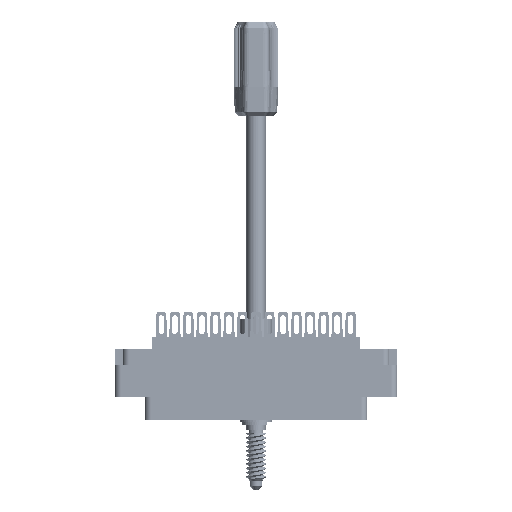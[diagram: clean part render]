
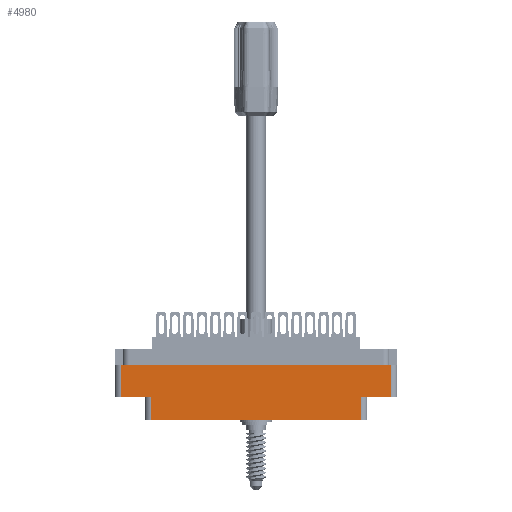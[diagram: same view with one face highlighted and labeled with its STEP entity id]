
A CAD part, front view. The second image highlights one B-rep face of the part: STEP entity #4980.
In plain terms, the highlighted planar face has unit normal (0, -1, 0).
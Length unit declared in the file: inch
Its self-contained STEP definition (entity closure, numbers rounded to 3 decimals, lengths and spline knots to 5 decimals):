
#68 = AXIS2_PLACEMENT_3D ( 'NONE', #38660, #51756, #12923 ) ;
#1185 = ORIENTED_EDGE ( 'NONE', *, *, #69164, .F. ) ;
#2698 = EDGE_CURVE ( 'NONE', #15390, #13735, #11628, .T. ) ;
#2727 = EDGE_CURVE ( 'NONE', #13735, #22982, #65832, .T. ) ;
#4980 = ADVANCED_FACE ( 'NONE', ( #72628 ), #77641, .T. ) ;
#5474 = CARTESIAN_POINT ( 'NONE',  ( 1.006, -0.617, -0.578 ) ) ;
#6226 = DIRECTION ( 'NONE',  ( 0., 0., -1. ) ) ;
#6946 = ORIENTED_EDGE ( 'NONE', *, *, #21479, .T. ) ;
#10073 = EDGE_CURVE ( 'NONE', #69673, #34776, #63557, .T. ) ;
#10220 = CARTESIAN_POINT ( 'NONE',  ( 0., -0.617, -0.578 ) ) ;
#10474 = ORIENTED_EDGE ( 'NONE', *, *, #2698, .T. ) ;
#11628 = LINE ( 'NONE', #51488, #83118 ) ;
#12923 = DIRECTION ( 'NONE',  ( 0., 0., -1. ) ) ;
#13735 = VERTEX_POINT ( 'NONE', #47508 ) ;
#15390 = VERTEX_POINT ( 'NONE', #29045 ) ;
#19813 = CARTESIAN_POINT ( 'NONE',  ( 0., -0.617, -0.578 ) ) ;
#21479 = EDGE_CURVE ( 'NONE', #49204, #60126, #30562, .T. ) ;
#21602 = ORIENTED_EDGE ( 'NONE', *, *, #44394, .F. ) ;
#22130 = LINE ( 'NONE', #24804, #57934 ) ;
#22982 = VERTEX_POINT ( 'NONE', #35612 ) ;
#24804 = CARTESIAN_POINT ( 'NONE',  ( 0., -0.617, -0.274 ) ) ;
#25062 = VECTOR ( 'NONE', #6226, 39.37008 ) ;
#27224 = DIRECTION ( 'NONE',  ( -1., 0., 0. ) ) ;
#28212 = CARTESIAN_POINT ( 'NONE',  ( -1.006, -0.617, -0.798 ) ) ;
#29045 = CARTESIAN_POINT ( 'NONE',  ( -1.006, -0.617, -0.798 ) ) ;
#29663 = CARTESIAN_POINT ( 'NONE',  ( -1.297, -0.617, -0.274 ) ) ;
#30562 = LINE ( 'NONE', #10220, #45898 ) ;
#31594 = CARTESIAN_POINT ( 'NONE',  ( 1.297, -0.617, -0.274 ) ) ;
#31770 = VECTOR ( 'NONE', #79518, 39.37008 ) ;
#34033 = ORIENTED_EDGE ( 'NONE', *, *, #10073, .T. ) ;
#34776 = VERTEX_POINT ( 'NONE', #31594 ) ;
#35612 = CARTESIAN_POINT ( 'NONE',  ( 1.006, -0.617, -0.578 ) ) ;
#36722 = EDGE_LOOP ( 'NONE', ( #6946, #54830, #10474, #54891, #1185, #34033, #21602, #52763 ) ) ;
#38660 = CARTESIAN_POINT ( 'NONE',  ( -1.359, -0.617, -0.798 ) ) ;
#42337 = VECTOR ( 'NONE', #58096, 39.37008 ) ;
#44394 = EDGE_CURVE ( 'NONE', #64825, #34776, #22130, .T. ) ;
#45319 = EDGE_CURVE ( 'NONE', #64825, #49204, #53655, .T. ) ;
#45898 = VECTOR ( 'NONE', #82438, 39.37008 ) ;
#47508 = CARTESIAN_POINT ( 'NONE',  ( 1.006, -0.617, -0.798 ) ) ;
#47764 = VECTOR ( 'NONE', #27224, 39.37008 ) ;
#49204 = VERTEX_POINT ( 'NONE', #56196 ) ;
#50012 = CARTESIAN_POINT ( 'NONE',  ( 1.297, -0.617, -0.798 ) ) ;
#51189 = DIRECTION ( 'NONE',  ( 1., 0., 0. ) ) ;
#51488 = CARTESIAN_POINT ( 'NONE',  ( -1.359, -0.617, -0.798 ) ) ;
#51756 = DIRECTION ( 'NONE',  ( 0., -1., 0. ) ) ;
#51900 = EDGE_CURVE ( 'NONE', #60126, #15390, #66513, .T. ) ;
#52763 = ORIENTED_EDGE ( 'NONE', *, *, #45319, .T. ) ;
#53655 = LINE ( 'NONE', #83906, #25062 ) ;
#54830 = ORIENTED_EDGE ( 'NONE', *, *, #51900, .T. ) ;
#54891 = ORIENTED_EDGE ( 'NONE', *, *, #2727, .T. ) ;
#56045 = DIRECTION ( 'NONE',  ( 0., 0., 1. ) ) ;
#56196 = CARTESIAN_POINT ( 'NONE',  ( -1.297, -0.617, -0.578 ) ) ;
#57925 = DIRECTION ( 'NONE',  ( 1., 0., 0. ) ) ;
#57934 = VECTOR ( 'NONE', #57925, 39.37008 ) ;
#58096 = DIRECTION ( 'NONE',  ( 0., 0., 1. ) ) ;
#60126 = VERTEX_POINT ( 'NONE', #78392 ) ;
#63557 = LINE ( 'NONE', #50012, #78738 ) ;
#64825 = VERTEX_POINT ( 'NONE', #29663 ) ;
#65832 = LINE ( 'NONE', #5474, #42337 ) ;
#66513 = LINE ( 'NONE', #28212, #31770 ) ;
#69164 = EDGE_CURVE ( 'NONE', #69673, #22982, #84369, .T. ) ;
#69673 = VERTEX_POINT ( 'NONE', #76102 ) ;
#72628 = FACE_OUTER_BOUND ( 'NONE', #36722, .T. ) ;
#76102 = CARTESIAN_POINT ( 'NONE',  ( 1.297, -0.617, -0.578 ) ) ;
#77641 = PLANE ( 'NONE',  #68 ) ;
#78392 = CARTESIAN_POINT ( 'NONE',  ( -1.006, -0.617, -0.578 ) ) ;
#78738 = VECTOR ( 'NONE', #56045, 39.37008 ) ;
#79518 = DIRECTION ( 'NONE',  ( 0., 0., -1. ) ) ;
#82438 = DIRECTION ( 'NONE',  ( 1., 0., 0. ) ) ;
#83118 = VECTOR ( 'NONE', #51189, 39.37008 ) ;
#83906 = CARTESIAN_POINT ( 'NONE',  ( -1.297, -0.617, -0.798 ) ) ;
#84369 = LINE ( 'NONE', #19813, #47764 ) ;
